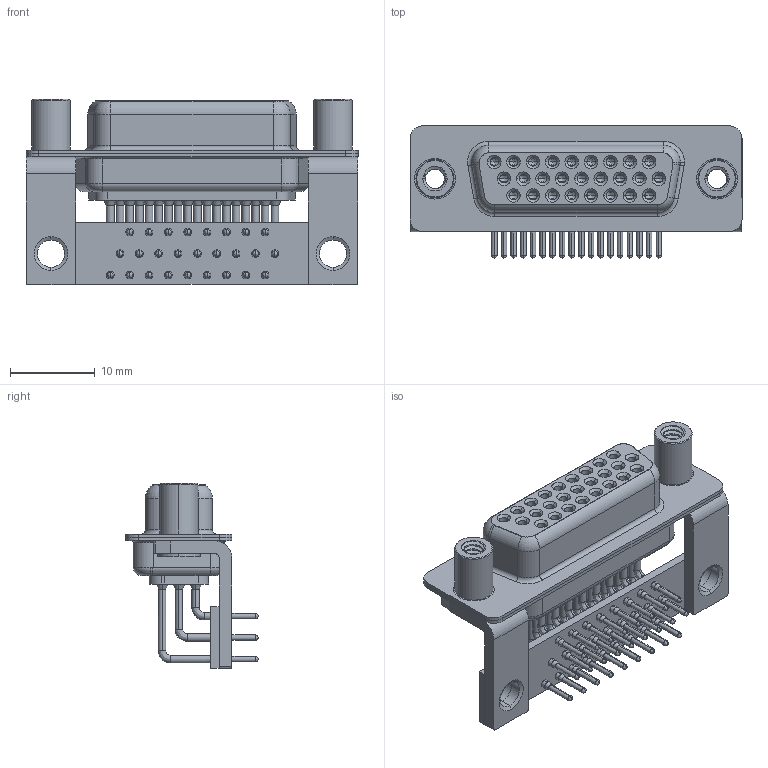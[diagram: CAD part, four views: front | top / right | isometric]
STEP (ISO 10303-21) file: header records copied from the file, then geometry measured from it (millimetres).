
FILE_DESCRIPTION (( 'STEP AP203' ), '1' );
FILE_NAME ('634-M26-263-BT6.STEP', '2018-09-27T22:41:36', ( '' ), ( '' ), 'SwSTEP 2.0', 'SolidWorks 2016', '' );
FILE_SCHEMA (( 'CONFIG_CONTROL_DESIGN' ));
Length unit declared in the file: millimetre
Products named in the file (10): 634M Contact Row 1; 634M Contact Row 2; 634M Contact Row 3; 634M Stabilizer Bracket; 634M 4-40 Threaded Standoff; 634M Stabilizer Board_26 Contacts; 634M Housing_26 Contacts; 634-M26-263-BT6; 634M Shell Front_26 Contacts; 634M Shell Rear_26 Contacts
Assembly tree (34 placements, depth 2):
  634-M26-263-BT6
    634M Housing_26 Contacts
    634M Shell Front_26 Contacts
    634M Shell Rear_26 Contacts
    634M Contact Row 1  x9
    634M Contact Row 2  x9
    634M Contact Row 3  x8
    634M Stabilizer Bracket  x2
    634M 4-40 Threaded Standoff  x2
    634M Stabilizer Board_26 Contacts
Bounding box: 39.2 x 15.6 x 21.9 mm (x, y, z)
Volume: 3190.3 mm3; surface area: 10090.2 mm2
Topology: 34 solids, 34 shells, 1809 faces, 4621 edges, 2919 vertices
Faces by surface type: cylinder 851, plane 485, cone 300, bspline 110, torus 63
Entity records: 27933 total; most frequent: CARTESIAN_POINT 6367, DIRECTION 4527, ORIENTED_EDGE 3888, EDGE_CURVE 1944, AXIS2_PLACEMENT_3D 1885, VERTEX_POINT 1245, CIRCLE 1052, EDGE_LOOP 1031
